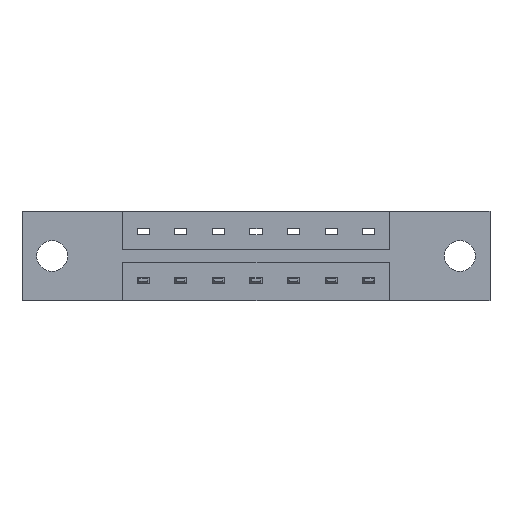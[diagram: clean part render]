
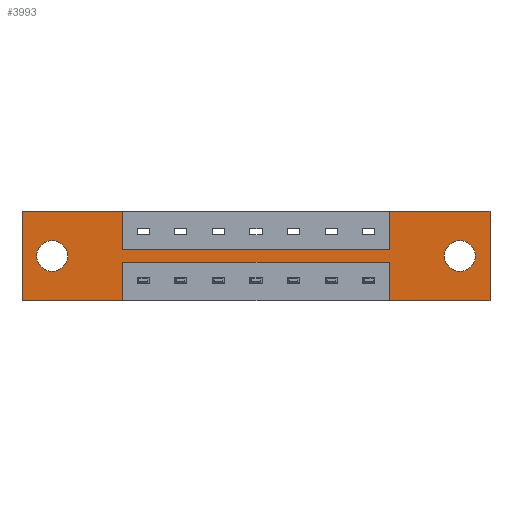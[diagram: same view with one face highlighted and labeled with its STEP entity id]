
A CAD part, front view. The second image highlights one B-rep face of the part: STEP entity #3993.
In plain terms, the highlighted planar face has unit normal (0, -1, 0).
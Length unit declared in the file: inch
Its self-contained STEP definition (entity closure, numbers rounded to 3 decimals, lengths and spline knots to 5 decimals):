
#128 = CARTESIAN_POINT ( 'NONE',  ( 0., 0., 0. ) ) ;
#139 = EDGE_CURVE ( 'NONE', #227, #7067, #4333, .T. ) ;
#227 = VERTEX_POINT ( 'NONE', #7815 ) ;
#334 = CARTESIAN_POINT ( 'NONE',  ( 1.5225, 0., -0.1585 ) ) ;
#450 = VERTEX_POINT ( 'NONE', #4577 ) ;
#588 = ORIENTED_EDGE ( 'NONE', *, *, #948, .F. ) ;
#639 = VECTOR ( 'NONE', #5257, 39.37008 ) ;
#677 = DIRECTION ( 'NONE',  ( 0., 0., -1. ) ) ;
#730 = ORIENTED_EDGE ( 'NONE', *, *, #139, .F. ) ;
#748 = CARTESIAN_POINT ( 'NONE',  ( 0.4175, 0., -0.1585 ) ) ;
#787 = CARTESIAN_POINT ( 'NONE',  ( 0., 0., -0.37 ) ) ;
#902 = DIRECTION ( 'NONE',  ( 0., 0., 1. ) ) ;
#943 = VERTEX_POINT ( 'NONE', #3648 ) ;
#948 = EDGE_CURVE ( 'NONE', #5781, #7916, #2216, .T. ) ;
#988 = CARTESIAN_POINT ( 'NONE',  ( 0.4175, 0., 0. ) ) ;
#1026 = DIRECTION ( 'NONE',  ( 1., 0., 0. ) ) ;
#1164 = CARTESIAN_POINT ( 'NONE',  ( 0.4175, 0., -0.1585 ) ) ;
#1215 = VECTOR ( 'NONE', #5522, 39.37008 ) ;
#1238 = LINE ( 'NONE', #3899, #6934 ) ;
#1330 = DIRECTION ( 'NONE',  ( 0., 0., 1. ) ) ;
#1340 = VERTEX_POINT ( 'NONE', #3690 ) ;
#1348 = ORIENTED_EDGE ( 'NONE', *, *, #1646, .T. ) ;
#1449 = DIRECTION ( 'NONE',  ( 0., 0., -1. ) ) ;
#1495 = CARTESIAN_POINT ( 'NONE',  ( 1.815, 0., -0.185 ) ) ;
#1646 = EDGE_CURVE ( 'NONE', #6318, #1340, #2083, .T. ) ;
#1735 = CARTESIAN_POINT ( 'NONE',  ( 1.94, 0., 0. ) ) ;
#1742 = EDGE_CURVE ( 'NONE', #450, #7409, #2776, .T. ) ;
#1759 = VECTOR ( 'NONE', #5517, 39.37008 ) ;
#1897 = LINE ( 'NONE', #4560, #639 ) ;
#1960 = VERTEX_POINT ( 'NONE', #7610 ) ;
#2049 = VECTOR ( 'NONE', #7845, 39.37008 ) ;
#2051 = ORIENTED_EDGE ( 'NONE', *, *, #4371, .F. ) ;
#2083 = CIRCLE ( 'NONE', #3326, 0.064 ) ;
#2091 = EDGE_CURVE ( 'NONE', #7409, #943, #1238, .T. ) ;
#2131 = CARTESIAN_POINT ( 'NONE',  ( 1.5225, 0., -0.2115 ) ) ;
#2188 = AXIS2_PLACEMENT_3D ( 'NONE', #4709, #5886, #677 ) ;
#2193 = EDGE_LOOP ( 'NONE', ( #4896, #2413, #4111, #2797, #730, #6540, #2051, #4985, #588, #2650, #4764, #4394 ) ) ;
#2194 = VECTOR ( 'NONE', #3228, 39.37008 ) ;
#2216 = LINE ( 'NONE', #7023, #3816 ) ;
#2391 = LINE ( 'NONE', #1164, #3293 ) ;
#2413 = ORIENTED_EDGE ( 'NONE', *, *, #3948, .F. ) ;
#2431 = LINE ( 'NONE', #7670, #2049 ) ;
#2479 = CARTESIAN_POINT ( 'NONE',  ( 1.94, 0., -0.37 ) ) ;
#2532 = CARTESIAN_POINT ( 'NONE',  ( 0., 0., -0.37 ) ) ;
#2599 = CIRCLE ( 'NONE', #2188, 0.064 ) ;
#2630 = CARTESIAN_POINT ( 'NONE',  ( 0., 0., 0. ) ) ;
#2650 = ORIENTED_EDGE ( 'NONE', *, *, #6498, .F. ) ;
#2739 = ORIENTED_EDGE ( 'NONE', *, *, #3446, .T. ) ;
#2776 = LINE ( 'NONE', #2131, #8219 ) ;
#2797 = ORIENTED_EDGE ( 'NONE', *, *, #4008, .F. ) ;
#2799 = AXIS2_PLACEMENT_3D ( 'NONE', #5445, #8565, #1330 ) ;
#2850 = LINE ( 'NONE', #7402, #1215 ) ;
#2891 = AXIS2_PLACEMENT_3D ( 'NONE', #4847, #6943, #902 ) ;
#3022 = ORIENTED_EDGE ( 'NONE', *, *, #4524, .T. ) ;
#3048 = LINE ( 'NONE', #4538, #2194 ) ;
#3180 = FACE_BOUND ( 'NONE', #3529, .T. ) ;
#3228 = DIRECTION ( 'NONE',  ( 1., 0., 0. ) ) ;
#3288 = CARTESIAN_POINT ( 'NONE',  ( 1.94, 0., 0. ) ) ;
#3293 = VECTOR ( 'NONE', #1026, 39.37008 ) ;
#3326 = AXIS2_PLACEMENT_3D ( 'NONE', #1495, #7516, #1449 ) ;
#3347 = DIRECTION ( 'NONE',  ( 0., 0., 1. ) ) ;
#3446 = EDGE_CURVE ( 'NONE', #8014, #5007, #5028, .T. ) ;
#3529 = EDGE_LOOP ( 'NONE', ( #3022, #1348 ) ) ;
#3648 = CARTESIAN_POINT ( 'NONE',  ( 0.4175, 0., -0.2115 ) ) ;
#3690 = CARTESIAN_POINT ( 'NONE',  ( 1.815, 0., -0.121 ) ) ;
#3693 = DIRECTION ( 'NONE',  ( 0., 0., -1. ) ) ;
#3800 = DIRECTION ( 'NONE',  ( 0., 0., 1. ) ) ;
#3816 = VECTOR ( 'NONE', #6319, 39.37008 ) ;
#3880 = DIRECTION ( 'NONE',  ( 0., 0., -1. ) ) ;
#3899 = CARTESIAN_POINT ( 'NONE',  ( 0.4175, 0., -0.2115 ) ) ;
#3948 = EDGE_CURVE ( 'NONE', #8335, #450, #2850, .T. ) ;
#3993 = ADVANCED_FACE ( 'NONE', ( #3180, #5238, #5196 ), #7767, .T. ) ;
#4008 = EDGE_CURVE ( 'NONE', #7067, #4813, #3048, .T. ) ;
#4111 = ORIENTED_EDGE ( 'NONE', *, *, #4369, .F. ) ;
#4246 = EDGE_CURVE ( 'NONE', #5007, #8014, #8188, .T. ) ;
#4333 = LINE ( 'NONE', #334, #5994 ) ;
#4369 = EDGE_CURVE ( 'NONE', #4813, #8335, #7801, .T. ) ;
#4371 = EDGE_CURVE ( 'NONE', #7052, #7661, #2431, .T. ) ;
#4394 = ORIENTED_EDGE ( 'NONE', *, *, #2091, .F. ) ;
#4430 = EDGE_CURVE ( 'NONE', #7661, #227, #2391, .T. ) ;
#4440 = CARTESIAN_POINT ( 'NONE',  ( 0., 0., -0.37 ) ) ;
#4524 = EDGE_CURVE ( 'NONE', #1340, #6318, #2599, .T. ) ;
#4538 = CARTESIAN_POINT ( 'NONE',  ( 0., 0., 0. ) ) ;
#4560 = CARTESIAN_POINT ( 'NONE',  ( 0.4175, 0., -0.2115 ) ) ;
#4577 = CARTESIAN_POINT ( 'NONE',  ( 1.5225, 0., -0.37 ) ) ;
#4709 = CARTESIAN_POINT ( 'NONE',  ( 1.815, 0., -0.185 ) ) ;
#4764 = ORIENTED_EDGE ( 'NONE', *, *, #4949, .F. ) ;
#4776 = ORIENTED_EDGE ( 'NONE', *, *, #4246, .T. ) ;
#4813 = VERTEX_POINT ( 'NONE', #3288 ) ;
#4847 = CARTESIAN_POINT ( 'NONE',  ( 0.125, 0., -0.185 ) ) ;
#4896 = ORIENTED_EDGE ( 'NONE', *, *, #1742, .F. ) ;
#4949 = EDGE_CURVE ( 'NONE', #943, #1960, #1897, .T. ) ;
#4985 = ORIENTED_EDGE ( 'NONE', *, *, #6451, .F. ) ;
#5007 = VERTEX_POINT ( 'NONE', #8173 ) ;
#5028 = CIRCLE ( 'NONE', #2799, 0.064 ) ;
#5196 = FACE_OUTER_BOUND ( 'NONE', #2193, .T. ) ;
#5238 = FACE_BOUND ( 'NONE', #6301, .T. ) ;
#5257 = DIRECTION ( 'NONE',  ( 0., 0., -1. ) ) ;
#5300 = DIRECTION ( 'NONE',  ( 1., 0., 0. ) ) ;
#5445 = CARTESIAN_POINT ( 'NONE',  ( 0.125, 0., -0.185 ) ) ;
#5517 = DIRECTION ( 'NONE',  ( -1., 0., 0. ) ) ;
#5522 = DIRECTION ( 'NONE',  ( -1., 0., 0. ) ) ;
#5727 = CARTESIAN_POINT ( 'NONE',  ( 0.125, 0., -0.249 ) ) ;
#5781 = VERTEX_POINT ( 'NONE', #4440 ) ;
#5886 = DIRECTION ( 'NONE',  ( 0., 1., 0. ) ) ;
#5994 = VECTOR ( 'NONE', #3800, 39.37008 ) ;
#6301 = EDGE_LOOP ( 'NONE', ( #4776, #2739 ) ) ;
#6318 = VERTEX_POINT ( 'NONE', #6610 ) ;
#6319 = DIRECTION ( 'NONE',  ( 0., 0., 1. ) ) ;
#6327 = CARTESIAN_POINT ( 'NONE',  ( 1.5225, 0., 0. ) ) ;
#6377 = AXIS2_PLACEMENT_3D ( 'NONE', #2532, #7895, #3880 ) ;
#6451 = EDGE_CURVE ( 'NONE', #7916, #7052, #8602, .T. ) ;
#6498 = EDGE_CURVE ( 'NONE', #1960, #5781, #8090, .T. ) ;
#6540 = ORIENTED_EDGE ( 'NONE', *, *, #4430, .F. ) ;
#6571 = DIRECTION ( 'NONE',  ( -1., 0., 0. ) ) ;
#6610 = CARTESIAN_POINT ( 'NONE',  ( 1.815, 0., -0.249 ) ) ;
#6650 = VECTOR ( 'NONE', #5300, 39.37008 ) ;
#6934 = VECTOR ( 'NONE', #6571, 39.37008 ) ;
#6943 = DIRECTION ( 'NONE',  ( 0., 1., 0. ) ) ;
#7023 = CARTESIAN_POINT ( 'NONE',  ( 0., 0., 0. ) ) ;
#7052 = VERTEX_POINT ( 'NONE', #988 ) ;
#7067 = VERTEX_POINT ( 'NONE', #6327 ) ;
#7402 = CARTESIAN_POINT ( 'NONE',  ( 0., 0., -0.37 ) ) ;
#7409 = VERTEX_POINT ( 'NONE', #7528 ) ;
#7516 = DIRECTION ( 'NONE',  ( 0., 1., 0. ) ) ;
#7528 = CARTESIAN_POINT ( 'NONE',  ( 1.5225, 0., -0.2115 ) ) ;
#7610 = CARTESIAN_POINT ( 'NONE',  ( 0.4175, 0., -0.37 ) ) ;
#7661 = VERTEX_POINT ( 'NONE', #748 ) ;
#7670 = CARTESIAN_POINT ( 'NONE',  ( 0.4175, 0., -0.1585 ) ) ;
#7767 = PLANE ( 'NONE',  #6377 ) ;
#7801 = LINE ( 'NONE', #1735, #8441 ) ;
#7815 = CARTESIAN_POINT ( 'NONE',  ( 1.5225, 0., -0.1585 ) ) ;
#7845 = DIRECTION ( 'NONE',  ( 0., 0., -1. ) ) ;
#7895 = DIRECTION ( 'NONE',  ( 0., -1., 0. ) ) ;
#7916 = VERTEX_POINT ( 'NONE', #128 ) ;
#8014 = VERTEX_POINT ( 'NONE', #5727 ) ;
#8090 = LINE ( 'NONE', #787, #1759 ) ;
#8173 = CARTESIAN_POINT ( 'NONE',  ( 0.125, 0., -0.121 ) ) ;
#8188 = CIRCLE ( 'NONE', #2891, 0.064 ) ;
#8219 = VECTOR ( 'NONE', #3347, 39.37008 ) ;
#8335 = VERTEX_POINT ( 'NONE', #2479 ) ;
#8441 = VECTOR ( 'NONE', #3693, 39.37008 ) ;
#8565 = DIRECTION ( 'NONE',  ( 0., 1., 0. ) ) ;
#8602 = LINE ( 'NONE', #2630, #6650 ) ;
